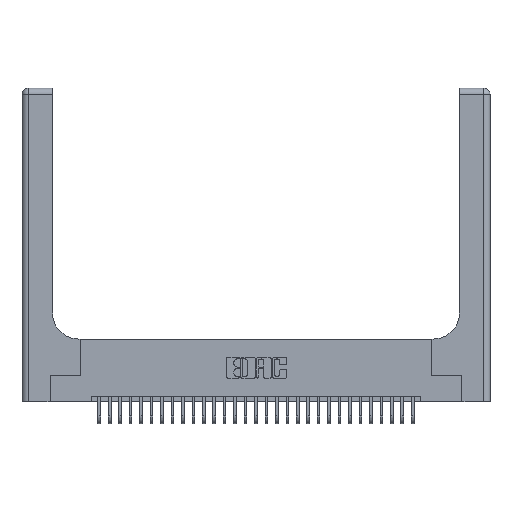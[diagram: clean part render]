
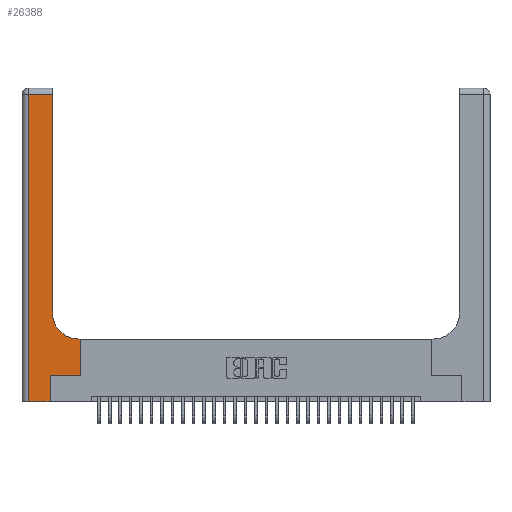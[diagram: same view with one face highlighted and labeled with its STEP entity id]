
A CAD part, top view. The second image highlights one B-rep face of the part: STEP entity #26388.
In plain terms, the highlighted planar face has unit normal (0, 0, 1).
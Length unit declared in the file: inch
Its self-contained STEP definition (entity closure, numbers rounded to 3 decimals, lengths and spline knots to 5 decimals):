
#22 = EDGE_CURVE ( 'NONE', #19567, #12301, #2982, .T. ) ;
#499 = DIRECTION ( 'NONE',  ( 1., 0., 0. ) ) ;
#2127 = LINE ( 'NONE', #3205, #25838 ) ;
#2229 = VECTOR ( 'NONE', #4927, 39.37008 ) ;
#2239 = DIRECTION ( 'NONE',  ( 0., 1., 0. ) ) ;
#2351 = CARTESIAN_POINT ( 'NONE',  ( 0.5585, 0.25, 0.37 ) ) ;
#2482 = ORIENTED_EDGE ( 'NONE', *, *, #17303, .T. ) ;
#2587 = CARTESIAN_POINT ( 'NONE',  ( 0.5415, 0.6, 0.37 ) ) ;
#2982 = LINE ( 'NONE', #9157, #17192 ) ;
#3205 = CARTESIAN_POINT ( 'NONE',  ( 0., 2.94, 0.37 ) ) ;
#3417 = CARTESIAN_POINT ( 'NONE',  ( 0.269, 0.25, 0.37 ) ) ;
#3452 = EDGE_CURVE ( 'NONE', #23091, #15335, #3950, .T. ) ;
#3535 = LINE ( 'NONE', #22329, #20927 ) ;
#3950 = LINE ( 'NONE', #4517, #28846 ) ;
#4416 = DIRECTION ( 'NONE',  ( -1., 0., 0. ) ) ;
#4517 = CARTESIAN_POINT ( 'NONE',  ( 0.269, 0.25, 0.37 ) ) ;
#4537 = VERTEX_POINT ( 'NONE', #31893 ) ;
#4927 = DIRECTION ( 'NONE',  ( 0., -1., 0. ) ) ;
#5793 = CARTESIAN_POINT ( 'NONE',  ( 0., 0., 0.37 ) ) ;
#6064 = CARTESIAN_POINT ( 'NONE',  ( 0.269, 0., 0.37 ) ) ;
#6956 = DIRECTION ( 'NONE',  ( 1., 0., 0. ) ) ;
#7682 = LINE ( 'NONE', #6064, #20315 ) ;
#8762 = LINE ( 'NONE', #5793, #21409 ) ;
#9157 = CARTESIAN_POINT ( 'NONE',  ( 0.2915, 0.6, 0.37 ) ) ;
#9797 = ORIENTED_EDGE ( 'NONE', *, *, #22, .T. ) ;
#10073 = CARTESIAN_POINT ( 'NONE',  ( 0.5585, 0.25, 0.37 ) ) ;
#11590 = VERTEX_POINT ( 'NONE', #25353 ) ;
#11676 = AXIS2_PLACEMENT_3D ( 'NONE', #11957, #29595, #6956 ) ;
#11957 = CARTESIAN_POINT ( 'NONE',  ( 0.5415, 0.85, 0.37 ) ) ;
#12255 = VERTEX_POINT ( 'NONE', #15167 ) ;
#12301 = VERTEX_POINT ( 'NONE', #2587 ) ;
#12957 = CARTESIAN_POINT ( 'NONE',  ( 0.2915, 0.85, 0.37 ) ) ;
#13799 = DIRECTION ( 'NONE',  ( 0., 1., 0. ) ) ;
#13813 = VERTEX_POINT ( 'NONE', #31342 ) ;
#13966 = ORIENTED_EDGE ( 'NONE', *, *, #16290, .T. ) ;
#14266 = CARTESIAN_POINT ( 'NONE',  ( 0.5585, 0.6, 0.37 ) ) ;
#14880 = ORIENTED_EDGE ( 'NONE', *, *, #3452, .T. ) ;
#15167 = CARTESIAN_POINT ( 'NONE',  ( 0.269, 0., 0.37 ) ) ;
#15335 = VERTEX_POINT ( 'NONE', #10073 ) ;
#16290 = EDGE_CURVE ( 'NONE', #13813, #12255, #8762, .T. ) ;
#16513 = LINE ( 'NONE', #2351, #31530 ) ;
#17192 = VECTOR ( 'NONE', #4416, 39.37008 ) ;
#17303 = EDGE_CURVE ( 'NONE', #26914, #4537, #3535, .T. ) ;
#18302 = DIRECTION ( 'NONE',  ( -1., 0., 0. ) ) ;
#18702 = EDGE_CURVE ( 'NONE', #15335, #19567, #16513, .T. ) ;
#19408 = CIRCLE ( 'NONE', #11676, 0.25 ) ;
#19567 = VERTEX_POINT ( 'NONE', #14266 ) ;
#19698 = EDGE_LOOP ( 'NONE', ( #2482, #25405, #32296, #13966, #23773, #14880, #28791, #9797, #26196 ) ) ;
#20050 = CARTESIAN_POINT ( 'NONE',  ( 0.06, 3., 0.37 ) ) ;
#20315 = VECTOR ( 'NONE', #13799, 39.37008 ) ;
#20927 = VECTOR ( 'NONE', #27510, 39.37008 ) ;
#21409 = VECTOR ( 'NONE', #499, 39.37008 ) ;
#22329 = CARTESIAN_POINT ( 'NONE',  ( 0.2915, 3., 0.37 ) ) ;
#22722 = EDGE_CURVE ( 'NONE', #12301, #26914, #19408, .T. ) ;
#23091 = VERTEX_POINT ( 'NONE', #3417 ) ;
#23269 = DIRECTION ( 'NONE',  ( -1., 0., 0. ) ) ;
#23773 = ORIENTED_EDGE ( 'NONE', *, *, #32279, .T. ) ;
#25353 = CARTESIAN_POINT ( 'NONE',  ( 0.06, 2.94, 0.37 ) ) ;
#25405 = ORIENTED_EDGE ( 'NONE', *, *, #32186, .T. ) ;
#25542 = LINE ( 'NONE', #20050, #2229 ) ;
#25838 = VECTOR ( 'NONE', #18302, 39.37008 ) ;
#25942 = AXIS2_PLACEMENT_3D ( 'NONE', #30635, #26336, #23269 ) ;
#26196 = ORIENTED_EDGE ( 'NONE', *, *, #22722, .T. ) ;
#26336 = DIRECTION ( 'NONE',  ( 0., 0., -1. ) ) ;
#26343 = DIRECTION ( 'NONE',  ( 1., 0., 0. ) ) ;
#26388 = ADVANCED_FACE ( 'NONE', ( #29051 ), #28101, .F. ) ;
#26914 = VERTEX_POINT ( 'NONE', #12957 ) ;
#27510 = DIRECTION ( 'NONE',  ( 0., 1., 0. ) ) ;
#28101 = PLANE ( 'NONE',  #25942 ) ;
#28791 = ORIENTED_EDGE ( 'NONE', *, *, #18702, .T. ) ;
#28846 = VECTOR ( 'NONE', #26343, 39.37008 ) ;
#29051 = FACE_OUTER_BOUND ( 'NONE', #19698, .T. ) ;
#29595 = DIRECTION ( 'NONE',  ( 0., 0., -1. ) ) ;
#30635 = CARTESIAN_POINT ( 'NONE',  ( 0., 3., 0.37 ) ) ;
#31044 = EDGE_CURVE ( 'NONE', #11590, #13813, #25542, .T. ) ;
#31342 = CARTESIAN_POINT ( 'NONE',  ( 0.06, 0., 0.37 ) ) ;
#31530 = VECTOR ( 'NONE', #2239, 39.37008 ) ;
#31893 = CARTESIAN_POINT ( 'NONE',  ( 0.2915, 2.94, 0.37 ) ) ;
#32186 = EDGE_CURVE ( 'NONE', #4537, #11590, #2127, .T. ) ;
#32279 = EDGE_CURVE ( 'NONE', #12255, #23091, #7682, .T. ) ;
#32296 = ORIENTED_EDGE ( 'NONE', *, *, #31044, .T. ) ;
